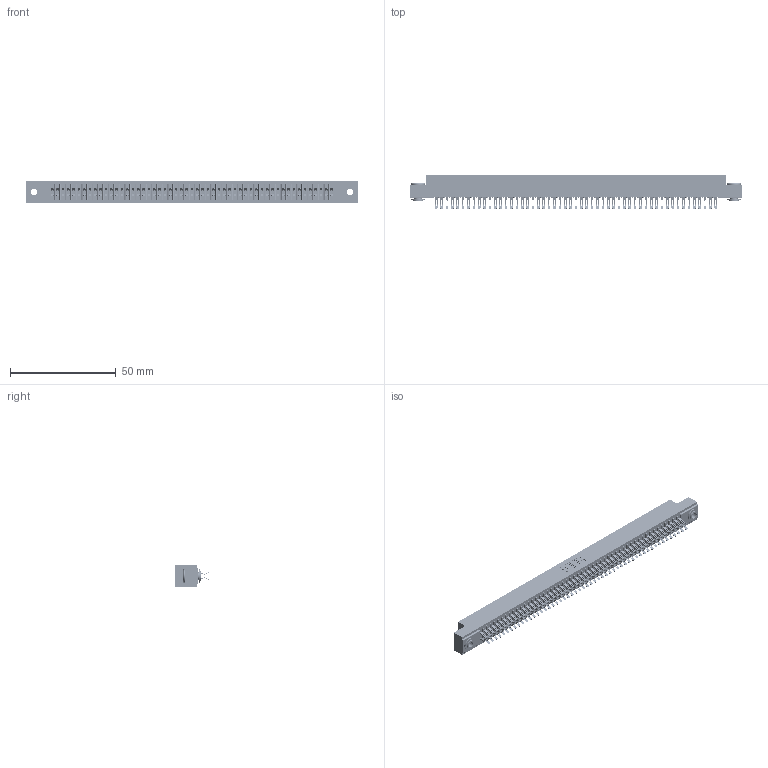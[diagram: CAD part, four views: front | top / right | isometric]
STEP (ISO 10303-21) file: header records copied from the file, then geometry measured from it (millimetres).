
FILE_DESCRIPTION (( 'STEP AP203' ), '1' );
FILE_NAME ('391-106-555-203.STEP', '2018-08-09T20:53:45', ( '' ), ( '' ), 'SwSTEP 2.0', 'SolidWorks 2016', '' );
FILE_SCHEMA (( 'CONFIG_CONTROL_DESIGN' ));
Length unit declared in the file: inch
Products named in the file (4): 391-106-555-203; 341 Part_.156 (3.96) Dia Mounting Holes; 341-292-001_341-292-155; 345-250-002_345-250-002-102
Assembly tree (109 placements, depth 2):
  391-106-555-203
    341 Part_.156 (3.96) Dia Mounting Holes
    341-292-001_341-292-155  x106
    345-250-002_345-250-002-102  x2
Bounding box: 156.84 x 16.31 x 10.16 mm (x, y, z)
Volume: 11727.9 mm3; surface area: 22275.2 mm2
Topology: 109 solids, 109 shells, 8436 faces, 25179 edges, 16390 vertices
Faces by surface type: plane 4544, cylinder 3672, sphere 108, torus 104, cone 8
Entity records: 64211 total; most frequent: CARTESIAN_POINT 10670, ORIENTED_EDGE 10586, DIRECTION 10353, EDGE_CURVE 5293, LINE 4263, VECTOR 4263, VERTEX_POINT 3346, AXIS2_PLACEMENT_3D 3045
